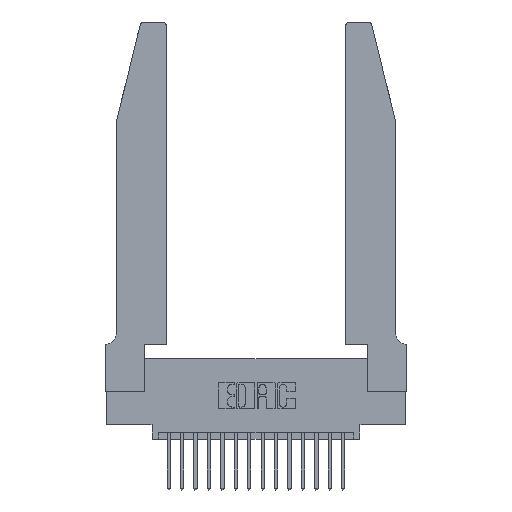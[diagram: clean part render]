
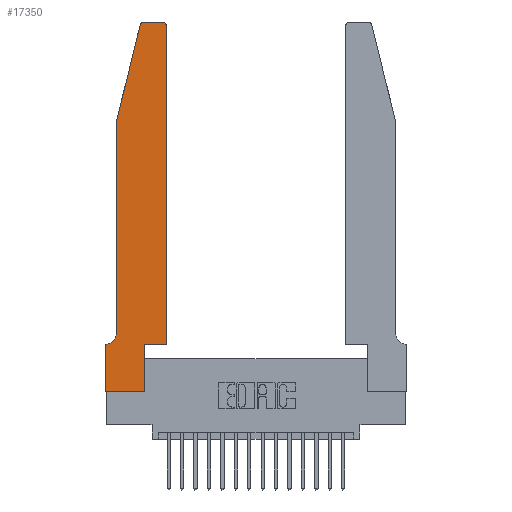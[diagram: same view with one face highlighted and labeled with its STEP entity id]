
A CAD part, top view. The second image highlights one B-rep face of the part: STEP entity #17350.
In plain terms, the highlighted planar face has unit normal (0, 0, 1).
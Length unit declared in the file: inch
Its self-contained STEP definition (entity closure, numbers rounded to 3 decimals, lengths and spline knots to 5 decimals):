
#122 = EDGE_CURVE ( 'NONE', #11330, #6666, #18211, .T. ) ;
#179 = CARTESIAN_POINT ( 'NONE',  ( 0.2865, 0.35, 0.37 ) ) ;
#199 = DIRECTION ( 'NONE',  ( 0., 0., -1. ) ) ;
#284 = ORIENTED_EDGE ( 'NONE', *, *, #7124, .T. ) ;
#580 = VERTEX_POINT ( 'NONE', #9553 ) ;
#634 = CARTESIAN_POINT ( 'NONE',  ( 0.0055, 0.35, 0.37 ) ) ;
#752 = ORIENTED_EDGE ( 'NONE', *, *, #122, .T. ) ;
#778 = EDGE_CURVE ( 'NONE', #3298, #9163, #3648, .T. ) ;
#1038 = VERTEX_POINT ( 'NONE', #15282 ) ;
#1241 = DIRECTION ( 'NONE',  ( 0., 0., 1. ) ) ;
#1277 = LINE ( 'NONE', #7610, #18162 ) ;
#1400 = EDGE_CURVE ( 'NONE', #2594, #1038, #10592, .T. ) ;
#1835 = ORIENTED_EDGE ( 'NONE', *, *, #10479, .T. ) ;
#1890 = EDGE_CURVE ( 'NONE', #3166, #14557, #1277, .T. ) ;
#2155 = CIRCLE ( 'NONE', #5734, 0.03 ) ;
#2235 = CARTESIAN_POINT ( 'NONE',  ( 0.2865, 0.35, 0.37 ) ) ;
#2308 = CARTESIAN_POINT ( 'NONE',  ( 0.4505, 0.35, 0.37 ) ) ;
#2446 = AXIS2_PLACEMENT_3D ( 'NONE', #4086, #1241, #11773 ) ;
#2594 = VERTEX_POINT ( 'NONE', #6636 ) ;
#2597 = LINE ( 'NONE', #3885, #4030 ) ;
#2629 = VERTEX_POINT ( 'NONE', #14671 ) ;
#2656 = ORIENTED_EDGE ( 'NONE', *, *, #4312, .T. ) ;
#2810 = ORIENTED_EDGE ( 'NONE', *, *, #18797, .T. ) ;
#2889 = CARTESIAN_POINT ( 'NONE',  ( 0., 0.35, 0.37 ) ) ;
#3166 = VERTEX_POINT ( 'NONE', #634 ) ;
#3298 = VERTEX_POINT ( 'NONE', #16173 ) ;
#3501 = CIRCLE ( 'NONE', #5999, 0.07 ) ;
#3648 = LINE ( 'NONE', #10278, #14827 ) ;
#3871 = CARTESIAN_POINT ( 'NONE',  ( 0.4505, 2.72, 0.37 ) ) ;
#3885 = CARTESIAN_POINT ( 'NONE',  ( 0.0755, 2., 0.37 ) ) ;
#3901 = DIRECTION ( 'NONE',  ( 0., 1., 0. ) ) ;
#4030 = VECTOR ( 'NONE', #19240, 39.37008 ) ;
#4086 = CARTESIAN_POINT ( 'NONE',  ( 0., 0.35, 0.37 ) ) ;
#4233 = VECTOR ( 'NONE', #4829, 39.37008 ) ;
#4312 = EDGE_CURVE ( 'NONE', #6666, #16579, #6804, .T. ) ;
#4341 = VECTOR ( 'NONE', #11699, 39.37008 ) ;
#4347 = PLANE ( 'NONE',  #2446 ) ;
#4394 = DIRECTION ( 'NONE',  ( 1., 0., 0. ) ) ;
#4829 = DIRECTION ( 'NONE',  ( 0., -1., 0. ) ) ;
#5653 = DIRECTION ( 'NONE',  ( 0., 0., 1. ) ) ;
#5734 = AXIS2_PLACEMENT_3D ( 'NONE', #7376, #5653, #4394 ) ;
#5999 = AXIS2_PLACEMENT_3D ( 'NONE', #6231, #199, #7832 ) ;
#6231 = CARTESIAN_POINT ( 'NONE',  ( 0.0055, 0.42, 0.37 ) ) ;
#6492 = CARTESIAN_POINT ( 'NONE',  ( 0.2605, 2.75, 0.37 ) ) ;
#6636 = CARTESIAN_POINT ( 'NONE',  ( 0.0755, 2., 0.37 ) ) ;
#6666 = VERTEX_POINT ( 'NONE', #7697 ) ;
#6804 = LINE ( 'NONE', #2235, #11143 ) ;
#7124 = EDGE_CURVE ( 'NONE', #16579, #3298, #7678, .T. ) ;
#7376 = CARTESIAN_POINT ( 'NONE',  ( 0.284, 2.72, 0.37 ) ) ;
#7610 = CARTESIAN_POINT ( 'NONE',  ( 0.0755, 0.35, 0.37 ) ) ;
#7678 = LINE ( 'NONE', #2308, #13855 ) ;
#7697 = CARTESIAN_POINT ( 'NONE',  ( 0.2865, 0., 0.37 ) ) ;
#7832 = DIRECTION ( 'NONE',  ( -1., 0., 0. ) ) ;
#7842 = ORIENTED_EDGE ( 'NONE', *, *, #778, .T. ) ;
#9163 = VERTEX_POINT ( 'NONE', #3871 ) ;
#9553 = CARTESIAN_POINT ( 'NONE',  ( 0.284, 2.75, 0.37 ) ) ;
#9645 = DIRECTION ( 'NONE',  ( 1., 0., 0. ) ) ;
#9931 = VECTOR ( 'NONE', #18603, 39.37008 ) ;
#10278 = CARTESIAN_POINT ( 'NONE',  ( 0.4505, 0.35, 0.37 ) ) ;
#10479 = EDGE_CURVE ( 'NONE', #1038, #3166, #3501, .T. ) ;
#10592 = LINE ( 'NONE', #19160, #4341 ) ;
#10874 = EDGE_CURVE ( 'NONE', #11326, #2594, #2597, .T. ) ;
#11132 = CARTESIAN_POINT ( 'NONE',  ( 0.4205, 2.72, 0.37 ) ) ;
#11143 = VECTOR ( 'NONE', #14667, 39.37008 ) ;
#11326 = VERTEX_POINT ( 'NONE', #12146 ) ;
#11330 = VERTEX_POINT ( 'NONE', #18152 ) ;
#11514 = DIRECTION ( 'NONE',  ( 1., 0., 0. ) ) ;
#11699 = DIRECTION ( 'NONE',  ( 0., -1., 0. ) ) ;
#11773 = DIRECTION ( 'NONE',  ( 1., 0., 0. ) ) ;
#12146 = CARTESIAN_POINT ( 'NONE',  ( 0.25487, 2.72718, 0.37 ) ) ;
#13855 = VECTOR ( 'NONE', #17719, 39.37008 ) ;
#14070 = CARTESIAN_POINT ( 'NONE',  ( 0., 0., 0.37 ) ) ;
#14253 = ORIENTED_EDGE ( 'NONE', *, *, #1890, .T. ) ;
#14263 = ORIENTED_EDGE ( 'NONE', *, *, #10874, .T. ) ;
#14339 = DIRECTION ( 'NONE',  ( 0., 0., 1. ) ) ;
#14557 = VERTEX_POINT ( 'NONE', #2889 ) ;
#14667 = DIRECTION ( 'NONE',  ( 0., 1., 0. ) ) ;
#14671 = CARTESIAN_POINT ( 'NONE',  ( 0.4205, 2.75, 0.37 ) ) ;
#14719 = CARTESIAN_POINT ( 'NONE',  ( 0., 0., 0.37 ) ) ;
#14827 = VECTOR ( 'NONE', #3901, 39.37008 ) ;
#14828 = AXIS2_PLACEMENT_3D ( 'NONE', #11132, #14339, #9645 ) ;
#15111 = VECTOR ( 'NONE', #11514, 39.37008 ) ;
#15282 = CARTESIAN_POINT ( 'NONE',  ( 0.0755, 0.42, 0.37 ) ) ;
#16125 = EDGE_LOOP ( 'NONE', ( #2810, #16334, #14263, #19512, #1835, #14253, #18895, #752, #2656, #284, #7842, #19409 ) ) ;
#16173 = CARTESIAN_POINT ( 'NONE',  ( 0.4505, 0.35, 0.37 ) ) ;
#16334 = ORIENTED_EDGE ( 'NONE', *, *, #16934, .T. ) ;
#16579 = VERTEX_POINT ( 'NONE', #179 ) ;
#16668 = DIRECTION ( 'NONE',  ( -1., 0., 0. ) ) ;
#16934 = EDGE_CURVE ( 'NONE', #580, #11326, #2155, .T. ) ;
#17350 = ADVANCED_FACE ( 'NONE', ( #17666 ), #4347, .T. ) ;
#17553 = EDGE_CURVE ( 'NONE', #14557, #11330, #18740, .T. ) ;
#17666 = FACE_OUTER_BOUND ( 'NONE', #16125, .T. ) ;
#17719 = DIRECTION ( 'NONE',  ( 1., 0., 0. ) ) ;
#17721 = CIRCLE ( 'NONE', #14828, 0.03 ) ;
#17989 = LINE ( 'NONE', #6492, #9931 ) ;
#18152 = CARTESIAN_POINT ( 'NONE',  ( 0., 0., 0.37 ) ) ;
#18162 = VECTOR ( 'NONE', #16668, 39.37008 ) ;
#18211 = LINE ( 'NONE', #14719, #15111 ) ;
#18603 = DIRECTION ( 'NONE',  ( -1., 0., 0. ) ) ;
#18740 = LINE ( 'NONE', #14070, #4233 ) ;
#18797 = EDGE_CURVE ( 'NONE', #2629, #580, #17989, .T. ) ;
#18799 = EDGE_CURVE ( 'NONE', #9163, #2629, #17721, .T. ) ;
#18895 = ORIENTED_EDGE ( 'NONE', *, *, #17553, .T. ) ;
#19160 = CARTESIAN_POINT ( 'NONE',  ( 0.0755, 2., 0.37 ) ) ;
#19240 = DIRECTION ( 'NONE',  ( -0.239, -0.971, 0. ) ) ;
#19409 = ORIENTED_EDGE ( 'NONE', *, *, #18799, .T. ) ;
#19512 = ORIENTED_EDGE ( 'NONE', *, *, #1400, .T. ) ;
